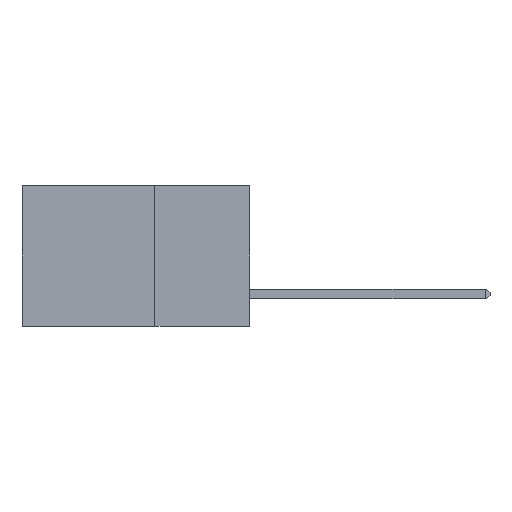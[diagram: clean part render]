
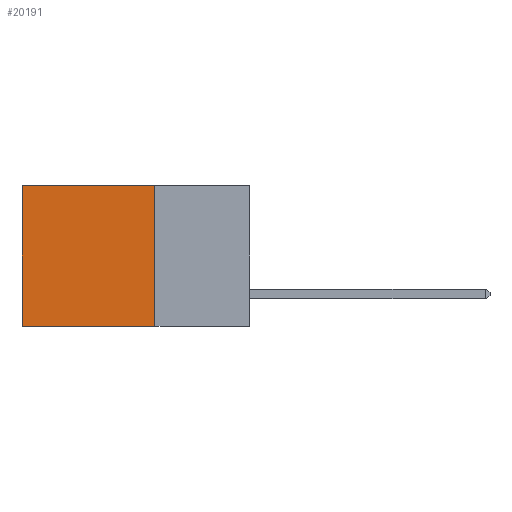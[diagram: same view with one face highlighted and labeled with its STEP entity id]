
A CAD part, left-side view. The second image highlights one B-rep face of the part: STEP entity #20191.
In plain terms, the highlighted planar face has unit normal (-1, 0, 0).
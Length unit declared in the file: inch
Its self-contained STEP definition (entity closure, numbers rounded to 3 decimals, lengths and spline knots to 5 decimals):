
#475 = CARTESIAN_POINT ( 'NONE',  ( 0.2875, 0.25, 0. ) ) ;
#2613 = ORIENTED_EDGE ( 'NONE', *, *, #18987, .T. ) ;
#3970 = ORIENTED_EDGE ( 'NONE', *, *, #11669, .T. ) ;
#5396 = VERTEX_POINT ( 'NONE', #16653 ) ;
#6171 = VECTOR ( 'NONE', #19973, 39.37008 ) ;
#6303 = EDGE_CURVE ( 'NONE', #24589, #5396, #6956, .T. ) ;
#6489 = VECTOR ( 'NONE', #9746, 39.37008 ) ;
#6956 = LINE ( 'NONE', #24882, #6171 ) ;
#7263 = LINE ( 'NONE', #22137, #6489 ) ;
#7393 = EDGE_CURVE ( 'NONE', #15480, #24589, #7263, .T. ) ;
#7741 = VECTOR ( 'NONE', #25578, 39.37008 ) ;
#9013 = FACE_OUTER_BOUND ( 'NONE', #22306, .T. ) ;
#9746 = DIRECTION ( 'NONE',  ( 0., 0., -1. ) ) ;
#10089 = PLANE ( 'NONE',  #25438 ) ;
#11669 = EDGE_CURVE ( 'NONE', #22402, #5396, #21019, .T. ) ;
#12605 = DIRECTION ( 'NONE',  ( 0., 0., -1. ) ) ;
#14132 = CARTESIAN_POINT ( 'NONE',  ( 0.2875, 0.6, 0. ) ) ;
#14325 = ORIENTED_EDGE ( 'NONE', *, *, #7393, .F. ) ;
#15480 = VERTEX_POINT ( 'NONE', #21684 ) ;
#16653 = CARTESIAN_POINT ( 'NONE',  ( 0.2875, 0.6, -0.37 ) ) ;
#18094 = DIRECTION ( 'NONE',  ( 0., 1., 0. ) ) ;
#18987 = EDGE_CURVE ( 'NONE', #15480, #22402, #31480, .T. ) ;
#19973 = DIRECTION ( 'NONE',  ( 0., 1., 0. ) ) ;
#20029 = VECTOR ( 'NONE', #18094, 39.37008 ) ;
#20191 = ADVANCED_FACE ( 'NONE', ( #9013 ), #10089, .F. ) ;
#21019 = LINE ( 'NONE', #23119, #7741 ) ;
#21684 = CARTESIAN_POINT ( 'NONE',  ( 0.2875, 0.25, 0. ) ) ;
#22137 = CARTESIAN_POINT ( 'NONE',  ( 0.2875, 0.25, 0. ) ) ;
#22306 = EDGE_LOOP ( 'NONE', ( #3970, #26985, #14325, #2613 ) ) ;
#22402 = VERTEX_POINT ( 'NONE', #14132 ) ;
#23119 = CARTESIAN_POINT ( 'NONE',  ( 0.2875, 0.6, 0. ) ) ;
#24589 = VERTEX_POINT ( 'NONE', #29888 ) ;
#24882 = CARTESIAN_POINT ( 'NONE',  ( 0.2875, 0.25, -0.37 ) ) ;
#24941 = CARTESIAN_POINT ( 'NONE',  ( 0.2875, 0.25, 0. ) ) ;
#25438 = AXIS2_PLACEMENT_3D ( 'NONE', #24941, #27384, #12605 ) ;
#25578 = DIRECTION ( 'NONE',  ( 0., 0., -1. ) ) ;
#26985 = ORIENTED_EDGE ( 'NONE', *, *, #6303, .F. ) ;
#27384 = DIRECTION ( 'NONE',  ( 1., 0., 0. ) ) ;
#29888 = CARTESIAN_POINT ( 'NONE',  ( 0.2875, 0.25, -0.37 ) ) ;
#31480 = LINE ( 'NONE', #475, #20029 ) ;
